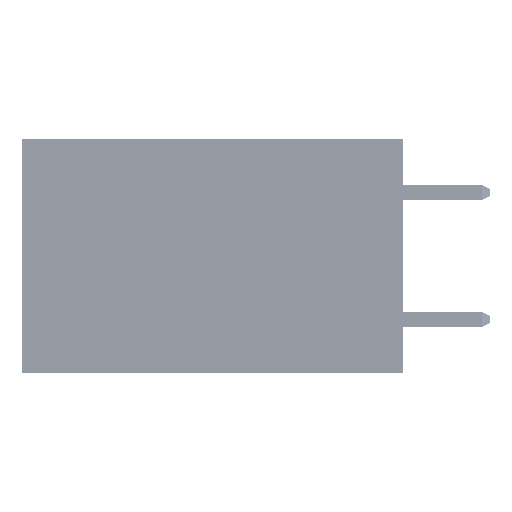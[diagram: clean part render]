
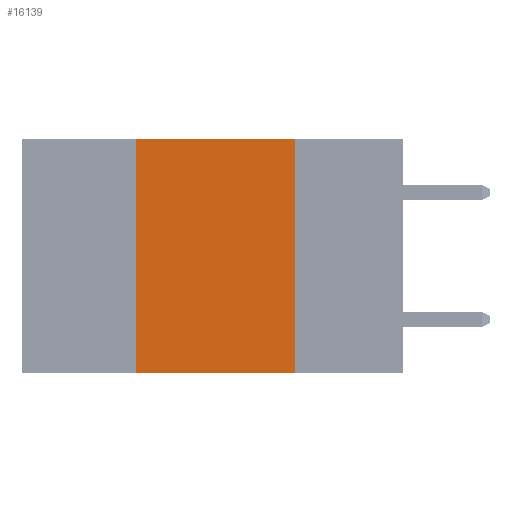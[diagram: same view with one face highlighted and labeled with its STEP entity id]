
A CAD part, left-side view. The second image highlights one B-rep face of the part: STEP entity #16139.
In plain terms, the highlighted planar face has unit normal (-1, 0, 0).
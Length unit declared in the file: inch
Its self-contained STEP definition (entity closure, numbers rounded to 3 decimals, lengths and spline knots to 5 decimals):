
#5068 = EDGE_CURVE ( 'NONE', #13503, #43230, #36917, .T. ) ;
#5707 = LINE ( 'NONE', #25879, #18538 ) ;
#6144 = DIRECTION ( 'NONE',  ( 1., 0., 0. ) ) ;
#6595 = VECTOR ( 'NONE', #49126, 39.37008 ) ;
#7293 = ORIENTED_EDGE ( 'NONE', *, *, #39198, .F. ) ;
#11165 = EDGE_LOOP ( 'NONE', ( #16636, #7293, #33040, #11425 ) ) ;
#11425 = ORIENTED_EDGE ( 'NONE', *, *, #37041, .T. ) ;
#13503 = VERTEX_POINT ( 'NONE', #47983 ) ;
#14988 = DIRECTION ( 'NONE',  ( 0., 0., -1. ) ) ;
#16139 = ADVANCED_FACE ( 'NONE', ( #49937 ), #26067, .F. ) ;
#16531 = VECTOR ( 'NONE', #14988, 39.37008 ) ;
#16636 = ORIENTED_EDGE ( 'NONE', *, *, #24471, .F. ) ;
#17298 = DIRECTION ( 'NONE',  ( 0., 0., -1. ) ) ;
#17459 = CARTESIAN_POINT ( 'NONE',  ( 0., 0.42, 0. ) ) ;
#18538 = VECTOR ( 'NONE', #21882, 39.37008 ) ;
#20215 = VECTOR ( 'NONE', #46126, 39.37008 ) ;
#21882 = DIRECTION ( 'NONE',  ( 0., -1., 0. ) ) ;
#22424 = LINE ( 'NONE', #38897, #16531 ) ;
#24471 = EDGE_CURVE ( 'NONE', #50315, #32063, #22424, .T. ) ;
#25879 = CARTESIAN_POINT ( 'NONE',  ( 0., 0.6, 0. ) ) ;
#26067 = PLANE ( 'NONE',  #32323 ) ;
#32063 = VERTEX_POINT ( 'NONE', #32377 ) ;
#32323 = AXIS2_PLACEMENT_3D ( 'NONE', #42240, #6144, #17298 ) ;
#32377 = CARTESIAN_POINT ( 'NONE',  ( 0., 0.17, -0.37 ) ) ;
#33040 = ORIENTED_EDGE ( 'NONE', *, *, #5068, .F. ) ;
#33689 = LINE ( 'NONE', #50121, #20215 ) ;
#36917 = LINE ( 'NONE', #37184, #6595 ) ;
#37041 = EDGE_CURVE ( 'NONE', #13503, #32063, #33689, .T. ) ;
#37184 = CARTESIAN_POINT ( 'NONE',  ( 0., 0.42, 0. ) ) ;
#38897 = CARTESIAN_POINT ( 'NONE',  ( 0., 0.17, 0. ) ) ;
#39198 = EDGE_CURVE ( 'NONE', #43230, #50315, #5707, .T. ) ;
#42240 = CARTESIAN_POINT ( 'NONE',  ( 0., 0.6, 0. ) ) ;
#43230 = VERTEX_POINT ( 'NONE', #17459 ) ;
#46126 = DIRECTION ( 'NONE',  ( 0., -1., 0. ) ) ;
#47983 = CARTESIAN_POINT ( 'NONE',  ( 0., 0.42, -0.37 ) ) ;
#49126 = DIRECTION ( 'NONE',  ( 0., 0., 1. ) ) ;
#49169 = CARTESIAN_POINT ( 'NONE',  ( 0., 0.17, 0. ) ) ;
#49937 = FACE_OUTER_BOUND ( 'NONE', #11165, .T. ) ;
#50121 = CARTESIAN_POINT ( 'NONE',  ( 0., 0.6, -0.37 ) ) ;
#50315 = VERTEX_POINT ( 'NONE', #49169 ) ;
